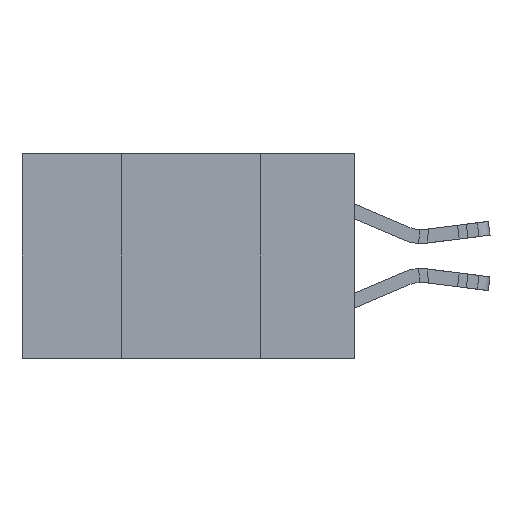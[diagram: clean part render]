
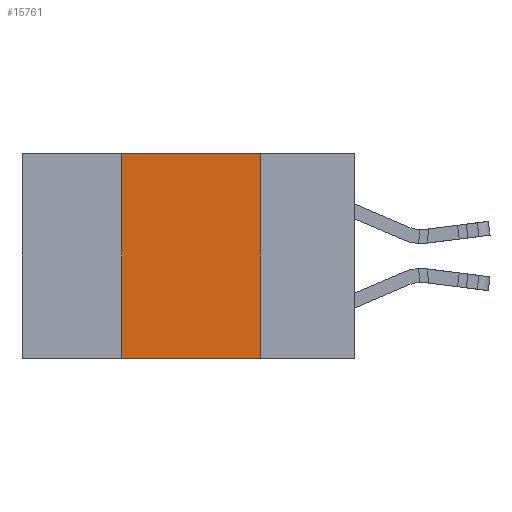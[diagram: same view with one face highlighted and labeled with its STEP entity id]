
A CAD part, left-side view. The second image highlights one B-rep face of the part: STEP entity #15761.
In plain terms, the highlighted planar face has unit normal (-1, 0, 0).
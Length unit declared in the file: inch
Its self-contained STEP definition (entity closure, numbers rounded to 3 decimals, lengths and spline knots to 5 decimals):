
#170 = CARTESIAN_POINT ( 'NONE',  ( 0., 0.42, -0.37 ) ) ;
#1499 = CARTESIAN_POINT ( 'NONE',  ( 0., 0.42, 0. ) ) ;
#3167 = CARTESIAN_POINT ( 'NONE',  ( 0., 0.6, -0.37 ) ) ;
#3672 = ORIENTED_EDGE ( 'NONE', *, *, #23819, .F. ) ;
#4123 = DIRECTION ( 'NONE',  ( 0., 0., 1. ) ) ;
#4469 = VECTOR ( 'NONE', #10337, 39.37008 ) ;
#4776 = EDGE_CURVE ( 'NONE', #12644, #23005, #24180, .T. ) ;
#7565 = ORIENTED_EDGE ( 'NONE', *, *, #10448, .F. ) ;
#8317 = DIRECTION ( 'NONE',  ( 0., -1., 0. ) ) ;
#9310 = FACE_OUTER_BOUND ( 'NONE', #18418, .T. ) ;
#10081 = VECTOR ( 'NONE', #8317, 39.37008 ) ;
#10337 = DIRECTION ( 'NONE',  ( 0., -1., 0. ) ) ;
#10448 = EDGE_CURVE ( 'NONE', #13733, #12644, #22853, .T. ) ;
#11260 = CARTESIAN_POINT ( 'NONE',  ( 0., 0.17, 0. ) ) ;
#11624 = DIRECTION ( 'NONE',  ( 0., 0., -1. ) ) ;
#11799 = CARTESIAN_POINT ( 'NONE',  ( 0., 0.6, 0. ) ) ;
#11943 = LINE ( 'NONE', #1499, #24006 ) ;
#12644 = VERTEX_POINT ( 'NONE', #23406 ) ;
#12954 = CARTESIAN_POINT ( 'NONE',  ( 0., 0.6, 0. ) ) ;
#13733 = VERTEX_POINT ( 'NONE', #28275 ) ;
#14182 = DIRECTION ( 'NONE',  ( 0., 0., -1. ) ) ;
#15761 = ADVANCED_FACE ( 'NONE', ( #9310 ), #26213, .F. ) ;
#18418 = EDGE_LOOP ( 'NONE', ( #24692, #7565, #3672, #28816 ) ) ;
#21666 = AXIS2_PLACEMENT_3D ( 'NONE', #11799, #28586, #14182 ) ;
#22103 = EDGE_CURVE ( 'NONE', #24115, #23005, #22850, .T. ) ;
#22675 = VECTOR ( 'NONE', #11624, 39.37008 ) ;
#22846 = CARTESIAN_POINT ( 'NONE',  ( 0., 0.17, -0.37 ) ) ;
#22850 = LINE ( 'NONE', #3167, #4469 ) ;
#22853 = LINE ( 'NONE', #12954, #10081 ) ;
#23005 = VERTEX_POINT ( 'NONE', #22846 ) ;
#23406 = CARTESIAN_POINT ( 'NONE',  ( 0., 0.17, 0. ) ) ;
#23819 = EDGE_CURVE ( 'NONE', #24115, #13733, #11943, .T. ) ;
#24006 = VECTOR ( 'NONE', #4123, 39.37008 ) ;
#24115 = VERTEX_POINT ( 'NONE', #170 ) ;
#24180 = LINE ( 'NONE', #11260, #22675 ) ;
#24692 = ORIENTED_EDGE ( 'NONE', *, *, #4776, .F. ) ;
#26213 = PLANE ( 'NONE',  #21666 ) ;
#28275 = CARTESIAN_POINT ( 'NONE',  ( 0., 0.42, 0. ) ) ;
#28586 = DIRECTION ( 'NONE',  ( 1., 0., 0. ) ) ;
#28816 = ORIENTED_EDGE ( 'NONE', *, *, #22103, .T. ) ;
